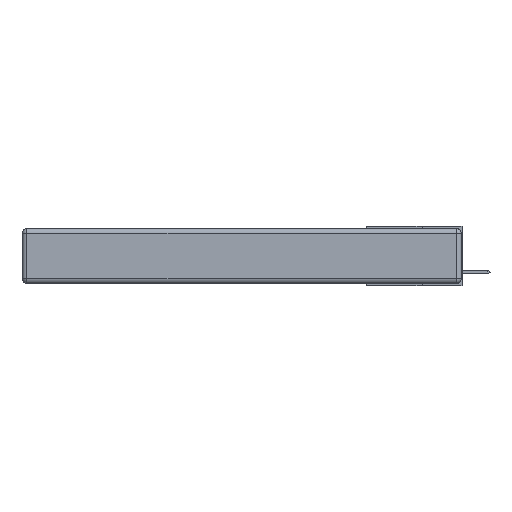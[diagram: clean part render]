
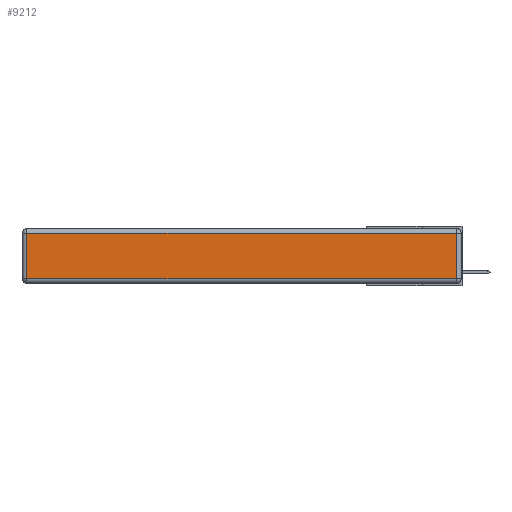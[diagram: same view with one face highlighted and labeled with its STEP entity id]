
A CAD part, left-side view. The second image highlights one B-rep face of the part: STEP entity #9212.
In plain terms, the highlighted planar face has unit normal (-1, 0, 0).
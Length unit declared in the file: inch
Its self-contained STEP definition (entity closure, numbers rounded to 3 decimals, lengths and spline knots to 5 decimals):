
#221 = CARTESIAN_POINT ( 'NONE',  ( 0., 2.75, -0.03 ) ) ;
#1519 = CARTESIAN_POINT ( 'NONE',  ( 0., 0.03, -0.343 ) ) ;
#1759 = CARTESIAN_POINT ( 'NONE',  ( 0., 2.72, -0.343 ) ) ;
#1937 = VECTOR ( 'NONE', #5789, 39.37008 ) ;
#2755 = EDGE_CURVE ( 'NONE', #5329, #8648, #17923, .T. ) ;
#3314 = VECTOR ( 'NONE', #7255, 39.37008 ) ;
#3472 = VECTOR ( 'NONE', #15997, 39.37008 ) ;
#3530 = VERTEX_POINT ( 'NONE', #15001 ) ;
#3663 = ORIENTED_EDGE ( 'NONE', *, *, #3753, .T. ) ;
#3753 = EDGE_CURVE ( 'NONE', #3530, #5329, #3916, .T. ) ;
#3916 = LINE ( 'NONE', #10033, #1937 ) ;
#4153 = DIRECTION ( 'NONE',  ( 0., 0., 1. ) ) ;
#5329 = VERTEX_POINT ( 'NONE', #10236 ) ;
#5789 = DIRECTION ( 'NONE',  ( 0., -1., 0. ) ) ;
#7045 = LINE ( 'NONE', #221, #3314 ) ;
#7255 = DIRECTION ( 'NONE',  ( 0., 1., 0. ) ) ;
#7645 = ORIENTED_EDGE ( 'NONE', *, *, #17981, .T. ) ;
#7796 = PLANE ( 'NONE',  #17789 ) ;
#8648 = VERTEX_POINT ( 'NONE', #10163 ) ;
#9121 = DIRECTION ( 'NONE',  ( -1., 0., 0. ) ) ;
#9212 = ADVANCED_FACE ( 'NONE', ( #16788 ), #7796, .T. ) ;
#9617 = CARTESIAN_POINT ( 'NONE',  ( 0., 2.72, -0.03 ) ) ;
#10033 = CARTESIAN_POINT ( 'NONE',  ( 0., 0., -0.313 ) ) ;
#10163 = CARTESIAN_POINT ( 'NONE',  ( 0., 0.03, -0.03 ) ) ;
#10236 = CARTESIAN_POINT ( 'NONE',  ( 0., 0.03, -0.313 ) ) ;
#10456 = CARTESIAN_POINT ( 'NONE',  ( 0., 0., -0.343 ) ) ;
#10840 = ORIENTED_EDGE ( 'NONE', *, *, #2755, .T. ) ;
#11134 = EDGE_LOOP ( 'NONE', ( #3663, #10840, #16183, #7645 ) ) ;
#12213 = LINE ( 'NONE', #1759, #3472 ) ;
#12635 = VERTEX_POINT ( 'NONE', #9617 ) ;
#13112 = VECTOR ( 'NONE', #4153, 39.37008 ) ;
#13288 = DIRECTION ( 'NONE',  ( 0., 0., 1. ) ) ;
#15001 = CARTESIAN_POINT ( 'NONE',  ( 0., 2.72, -0.313 ) ) ;
#15599 = EDGE_CURVE ( 'NONE', #8648, #12635, #7045, .T. ) ;
#15997 = DIRECTION ( 'NONE',  ( 0., 0., -1. ) ) ;
#16183 = ORIENTED_EDGE ( 'NONE', *, *, #15599, .T. ) ;
#16788 = FACE_OUTER_BOUND ( 'NONE', #11134, .T. ) ;
#17789 = AXIS2_PLACEMENT_3D ( 'NONE', #10456, #9121, #13288 ) ;
#17923 = LINE ( 'NONE', #1519, #13112 ) ;
#17981 = EDGE_CURVE ( 'NONE', #12635, #3530, #12213, .T. ) ;
